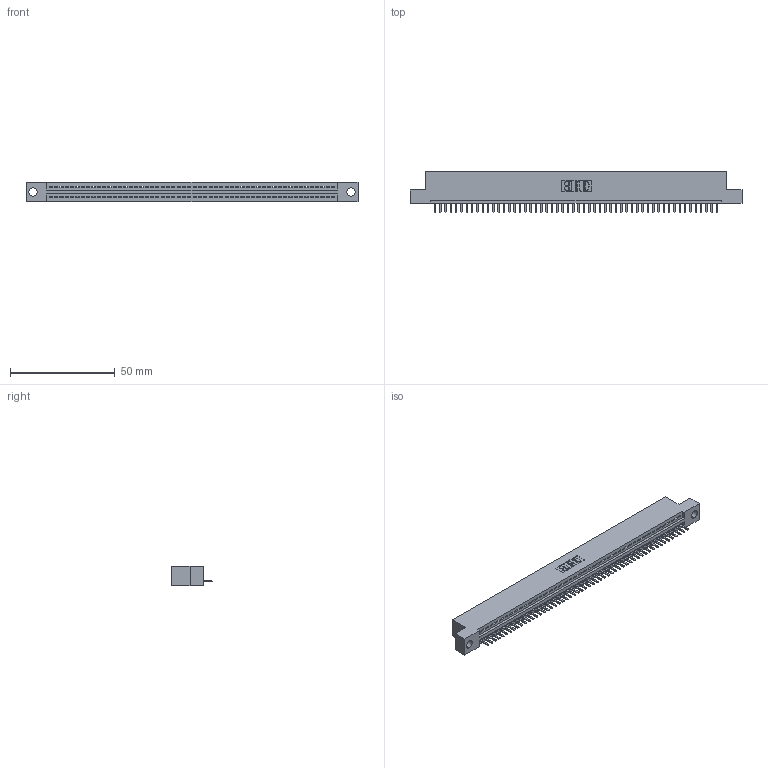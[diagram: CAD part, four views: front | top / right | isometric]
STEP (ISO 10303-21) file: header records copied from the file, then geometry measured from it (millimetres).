
FILE_DESCRIPTION (( 'STEP AP203' ), '1' );
FILE_NAME ('395-054-520-104.STEP', '2018-11-21T06:00:01', ( '' ), ( '' ), 'SwSTEP 2.0', 'SolidWorks 2016', '' );
FILE_SCHEMA (( 'CONFIG_CONTROL_DESIGN' ));
Length unit declared in the file: inch
Products named in the file (3): 395-054-520-104; 345 Part_Flush Mounting Lugs - 0.156 Dia-TH; 345-292-001_345-293-120
Assembly tree (55 placements, depth 2):
  395-054-520-104
    345 Part_Flush Mounting Lugs - 0.156 Dia-TH
    345-292-001_345-293-120  x54
Bounding box: 158.37 x 19.68 x 9.4 mm (x, y, z)
Volume: 14897.2 mm3; surface area: 19260.7 mm2
Topology: 55 solids, 55 shells, 3474 faces, 10277 edges, 6706 vertices
Faces by surface type: plane 2348, cylinder 1126
Entity records: 39143 total; most frequent: CARTESIAN_POINT 6798, ORIENTED_EDGE 6774, DIRECTION 5907, EDGE_CURVE 3387, LINE 3035, VECTOR 3035, VERTEX_POINT 2254, AXIS2_PLACEMENT_3D 1436
